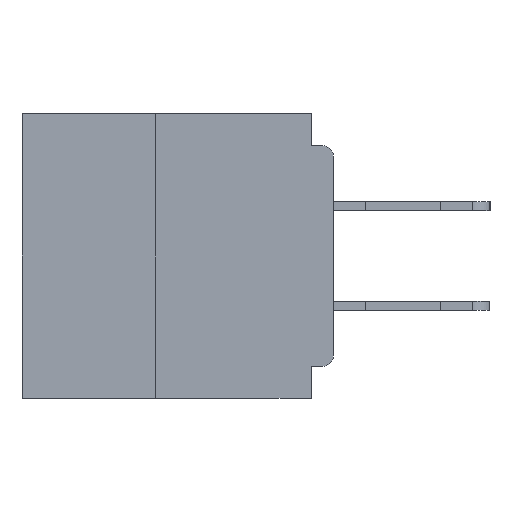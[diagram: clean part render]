
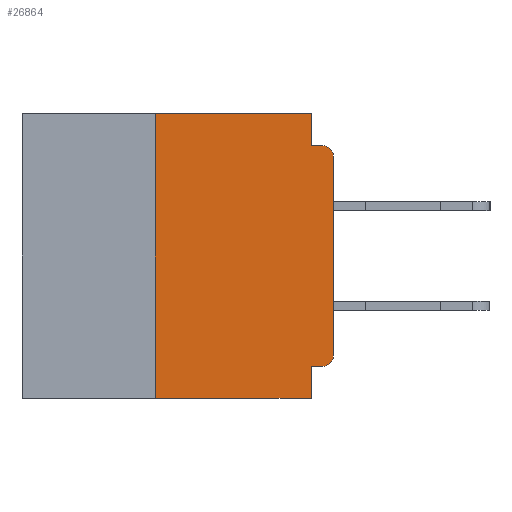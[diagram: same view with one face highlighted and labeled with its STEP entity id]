
A CAD part, left-side view. The second image highlights one B-rep face of the part: STEP entity #26864.
In plain terms, the highlighted planar face has unit normal (-1, 0, 0).
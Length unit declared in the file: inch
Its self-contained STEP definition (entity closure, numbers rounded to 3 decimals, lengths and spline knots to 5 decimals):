
#71 = VECTOR ( 'NONE', #26572, 39.37008 ) ;
#559 = CARTESIAN_POINT ( 'NONE',  ( 0., 0.25, -0.4 ) ) ;
#878 = ORIENTED_EDGE ( 'NONE', *, *, #25033, .T. ) ;
#1036 = FACE_OUTER_BOUND ( 'NONE', #14438, .T. ) ;
#1251 = DIRECTION ( 'NONE',  ( 0., -1., 0. ) ) ;
#1308 = CARTESIAN_POINT ( 'NONE',  ( 0., 0., -0.045 ) ) ;
#1532 = AXIS2_PLACEMENT_3D ( 'NONE', #15490, #42269, #19415 ) ;
#1764 = EDGE_CURVE ( 'NONE', #43047, #40538, #44378, .T. ) ;
#2504 = LINE ( 'NONE', #18735, #23121 ) ;
#4298 = CARTESIAN_POINT ( 'NONE',  ( 0., 0., -0.34 ) ) ;
#4609 = ORIENTED_EDGE ( 'NONE', *, *, #1764, .F. ) ;
#5644 = CARTESIAN_POINT ( 'NONE',  ( 0., 0.031, -0.4 ) ) ;
#5885 = CARTESIAN_POINT ( 'NONE',  ( 0., 0.015, -0.34 ) ) ;
#6228 = LINE ( 'NONE', #6586, #25547 ) ;
#6550 = CIRCLE ( 'NONE', #35744, 0.015 ) ;
#6578 = ORIENTED_EDGE ( 'NONE', *, *, #15765, .F. ) ;
#6586 = CARTESIAN_POINT ( 'NONE',  ( 0., 0.437, -0.4 ) ) ;
#8514 = VECTOR ( 'NONE', #20025, 39.37008 ) ;
#8738 = CARTESIAN_POINT ( 'NONE',  ( 0., 0., -0.355 ) ) ;
#9358 = VERTEX_POINT ( 'NONE', #559 ) ;
#9817 = DIRECTION ( 'NONE',  ( 0., 0., -1. ) ) ;
#9881 = LINE ( 'NONE', #8738, #49392 ) ;
#10936 = CARTESIAN_POINT ( 'NONE',  ( 0., 0.031, -0.4 ) ) ;
#11998 = CARTESIAN_POINT ( 'NONE',  ( 0., 0.015, -0.355 ) ) ;
#12429 = CARTESIAN_POINT ( 'NONE',  ( 0., 0.031, -0.355 ) ) ;
#12697 = DIRECTION ( 'NONE',  ( 0., 0., -1. ) ) ;
#14438 = EDGE_LOOP ( 'NONE', ( #18724, #23203, #4609, #46671, #18868, #22608, #878, #32270, #6578, #37420 ) ) ;
#14459 = DIRECTION ( 'NONE',  ( 0., -1., 0. ) ) ;
#14745 = EDGE_CURVE ( 'NONE', #28026, #17933, #47706, .T. ) ;
#15490 = CARTESIAN_POINT ( 'NONE',  ( 0., 0.015, -0.06 ) ) ;
#15765 = EDGE_CURVE ( 'NONE', #29147, #28026, #9881, .T. ) ;
#17933 = VERTEX_POINT ( 'NONE', #10936 ) ;
#18318 = DIRECTION ( 'NONE',  ( 0., -1., 0. ) ) ;
#18724 = ORIENTED_EDGE ( 'NONE', *, *, #30270, .T. ) ;
#18735 = CARTESIAN_POINT ( 'NONE',  ( 0., 0.25, -0.4 ) ) ;
#18846 = LINE ( 'NONE', #35197, #8514 ) ;
#18868 = ORIENTED_EDGE ( 'NONE', *, *, #42501, .F. ) ;
#19415 = DIRECTION ( 'NONE',  ( 0., 0., -1. ) ) ;
#20025 = DIRECTION ( 'NONE',  ( 0., 0., -1. ) ) ;
#21616 = CARTESIAN_POINT ( 'NONE',  ( 0., 0.015, -0.045 ) ) ;
#22608 = ORIENTED_EDGE ( 'NONE', *, *, #30206, .F. ) ;
#23121 = VECTOR ( 'NONE', #45409, 39.37008 ) ;
#23203 = ORIENTED_EDGE ( 'NONE', *, *, #47438, .T. ) ;
#25015 = CARTESIAN_POINT ( 'NONE',  ( 0., 0., -0.06 ) ) ;
#25033 = EDGE_CURVE ( 'NONE', #9358, #17933, #6228, .T. ) ;
#25487 = AXIS2_PLACEMENT_3D ( 'NONE', #31865, #35707, #12697 ) ;
#25547 = VECTOR ( 'NONE', #18318, 39.37008 ) ;
#26181 = VERTEX_POINT ( 'NONE', #25015 ) ;
#26572 = DIRECTION ( 'NONE',  ( 0., 0., 1. ) ) ;
#26851 = VECTOR ( 'NONE', #14459, 39.37008 ) ;
#26864 = ADVANCED_FACE ( 'NONE', ( #1036 ), #28018, .F. ) ;
#27009 = EDGE_CURVE ( 'NONE', #29147, #46478, #6550, .T. ) ;
#28018 = PLANE ( 'NONE',  #25487 ) ;
#28026 = VERTEX_POINT ( 'NONE', #12429 ) ;
#28850 = CARTESIAN_POINT ( 'NONE',  ( 0., 0.25, 0. ) ) ;
#29147 = VERTEX_POINT ( 'NONE', #11998 ) ;
#29185 = CARTESIAN_POINT ( 'NONE',  ( 0., 0.031, -0.045 ) ) ;
#30206 = EDGE_CURVE ( 'NONE', #9358, #32917, #2504, .T. ) ;
#30270 = EDGE_CURVE ( 'NONE', #46478, #26181, #30901, .T. ) ;
#30901 = LINE ( 'NONE', #45567, #71 ) ;
#30955 = CARTESIAN_POINT ( 'NONE',  ( 0., 0.031, 0. ) ) ;
#31865 = CARTESIAN_POINT ( 'NONE',  ( 0., 0.437, 0. ) ) ;
#32270 = ORIENTED_EDGE ( 'NONE', *, *, #14745, .F. ) ;
#32752 = EDGE_CURVE ( 'NONE', #40809, #43047, #18846, .T. ) ;
#32874 = DIRECTION ( 'NONE',  ( -1., 0., 0. ) ) ;
#32917 = VERTEX_POINT ( 'NONE', #28850 ) ;
#35197 = CARTESIAN_POINT ( 'NONE',  ( 0., 0.031, 0. ) ) ;
#35337 = CIRCLE ( 'NONE', #1532, 0.015 ) ;
#35619 = DIRECTION ( 'NONE',  ( 0., 1., 0. ) ) ;
#35707 = DIRECTION ( 'NONE',  ( 1., 0., 0. ) ) ;
#35744 = AXIS2_PLACEMENT_3D ( 'NONE', #5885, #32874, #9817 ) ;
#37420 = ORIENTED_EDGE ( 'NONE', *, *, #27009, .T. ) ;
#40538 = VERTEX_POINT ( 'NONE', #21616 ) ;
#40809 = VERTEX_POINT ( 'NONE', #30955 ) ;
#42269 = DIRECTION ( 'NONE',  ( -1., 0., 0. ) ) ;
#42501 = EDGE_CURVE ( 'NONE', #32917, #40809, #47116, .T. ) ;
#43047 = VERTEX_POINT ( 'NONE', #29185 ) ;
#43160 = VECTOR ( 'NONE', #1251, 39.37008 ) ;
#44378 = LINE ( 'NONE', #1308, #43160 ) ;
#45409 = DIRECTION ( 'NONE',  ( 0., 0., 1. ) ) ;
#45567 = CARTESIAN_POINT ( 'NONE',  ( 0., 0., 0. ) ) ;
#46478 = VERTEX_POINT ( 'NONE', #4298 ) ;
#46534 = VECTOR ( 'NONE', #47744, 39.37008 ) ;
#46671 = ORIENTED_EDGE ( 'NONE', *, *, #32752, .F. ) ;
#47116 = LINE ( 'NONE', #48865, #26851 ) ;
#47438 = EDGE_CURVE ( 'NONE', #26181, #40538, #35337, .T. ) ;
#47706 = LINE ( 'NONE', #5644, #46534 ) ;
#47744 = DIRECTION ( 'NONE',  ( 0., 0., -1. ) ) ;
#48865 = CARTESIAN_POINT ( 'NONE',  ( 0., 0.437, 0. ) ) ;
#49392 = VECTOR ( 'NONE', #35619, 39.37008 ) ;
